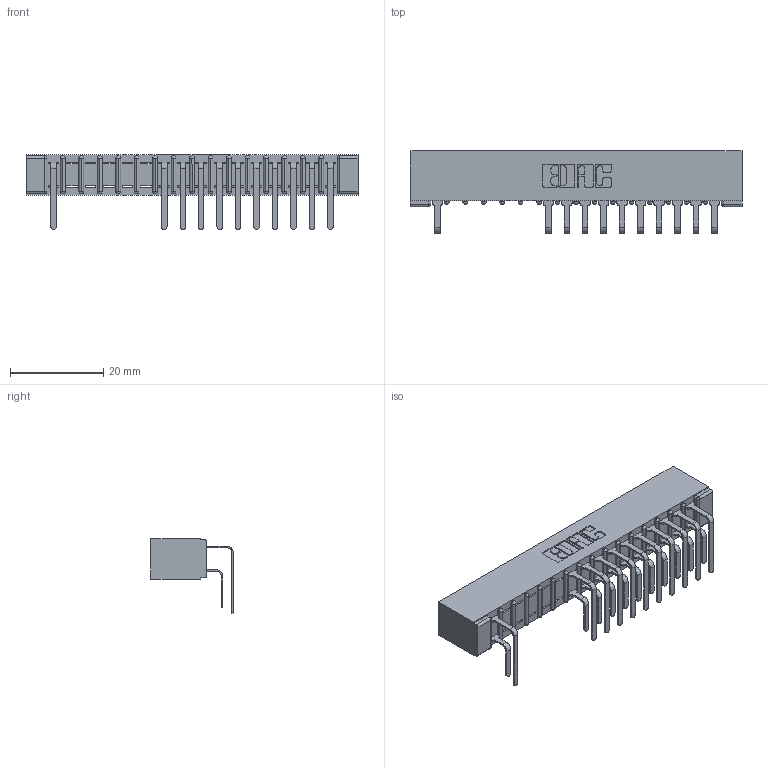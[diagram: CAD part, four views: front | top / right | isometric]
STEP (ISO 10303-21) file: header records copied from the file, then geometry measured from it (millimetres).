
FILE_DESCRIPTION (( 'STEP AP203' ), '1' );
FILE_NAME ('307-016-559-101.STEP', '2018-08-03T03:08:14', ( '' ), ( '' ), 'SwSTEP 2.0', 'SolidWorks 2016', '' );
FILE_SCHEMA (( 'CONFIG_CONTROL_DESIGN' ));
Length unit declared in the file: inch
Products named in the file (4): 307 Part_No Mounting Lugs; 307-290-001_558 559 - 1 (Single); 307-290-001_559 - 2 (Single); 307-016-559-101
Assembly tree (23 placements, depth 2):
  307-016-559-101
    307 Part_No Mounting Lugs
    307-290-001_558 559 - 1 (Single)  x11
    307-290-001_559 - 2 (Single)  x11
Bounding box: 71.27 x 17.69 x 16.08 mm (x, y, z)
Volume: 4863.8 mm3; surface area: 8532.9 mm2
Topology: 23 solids, 23 shells, 1327 faces, 3743 edges, 2418 vertices
Faces by surface type: plane 852, cylinder 441, sphere 34
Entity records: 18283 total; most frequent: CARTESIAN_POINT 3040, ORIENTED_EDGE 3018, DIRECTION 2977, EDGE_CURVE 1509, LINE 1147, VECTOR 1147, VERTEX_POINT 978, AXIS2_PLACEMENT_3D 915
